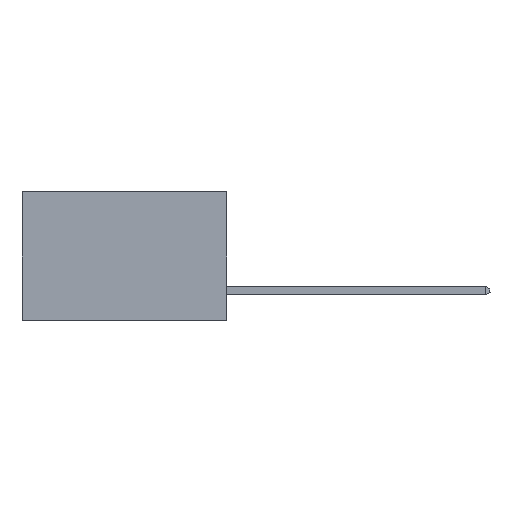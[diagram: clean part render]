
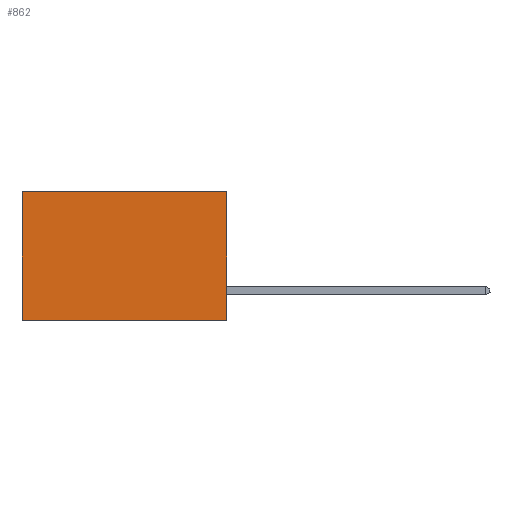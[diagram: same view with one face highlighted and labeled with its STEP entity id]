
A CAD part, left-side view. The second image highlights one B-rep face of the part: STEP entity #862.
In plain terms, the highlighted planar face has unit normal (-1, 0, 0).
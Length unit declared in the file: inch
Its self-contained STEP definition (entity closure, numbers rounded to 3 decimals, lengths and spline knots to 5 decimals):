
#36 = ORIENTED_EDGE ( 'NONE', *, *, #1651, .F. ) ;
#275 = CARTESIAN_POINT ( 'NONE',  ( 0.277, 0.59, 0. ) ) ;
#862 = ADVANCED_FACE ( 'NONE', ( #5057 ), #7052, .F. ) ;
#1097 = VERTEX_POINT ( 'NONE', #275 ) ;
#1651 = EDGE_CURVE ( 'NONE', #5266, #9212, #3417, .T. ) ;
#1673 = EDGE_CURVE ( 'NONE', #7320, #5266, #9046, .T. ) ;
#1677 = CARTESIAN_POINT ( 'NONE',  ( 0.277, 0.59, -0.37 ) ) ;
#1710 = CARTESIAN_POINT ( 'NONE',  ( 0.277, 0.59, -0.37 ) ) ;
#1860 = CARTESIAN_POINT ( 'NONE',  ( 0.277, 0., -0.37 ) ) ;
#2819 = DIRECTION ( 'NONE',  ( 1., 0., 0. ) ) ;
#2960 = CARTESIAN_POINT ( 'NONE',  ( 0.277, 0., 0. ) ) ;
#3206 = CARTESIAN_POINT ( 'NONE',  ( 0.277, 0., -0.37 ) ) ;
#3212 = CARTESIAN_POINT ( 'NONE',  ( 0.277, 0., 0. ) ) ;
#3417 = LINE ( 'NONE', #1860, #7367 ) ;
#4752 = ORIENTED_EDGE ( 'NONE', *, *, #1673, .F. ) ;
#5057 = FACE_OUTER_BOUND ( 'NONE', #7491, .T. ) ;
#5266 = VERTEX_POINT ( 'NONE', #9908 ) ;
#6679 = DIRECTION ( 'NONE',  ( 0., 1., 0. ) ) ;
#6846 = ORIENTED_EDGE ( 'NONE', *, *, #8831, .T. ) ;
#6894 = VECTOR ( 'NONE', #8727, 39.37008 ) ;
#7052 = PLANE ( 'NONE',  #7210 ) ;
#7128 = VECTOR ( 'NONE', #7342, 39.37008 ) ;
#7210 = AXIS2_PLACEMENT_3D ( 'NONE', #9140, #2819, #9097 ) ;
#7320 = VERTEX_POINT ( 'NONE', #2960 ) ;
#7342 = DIRECTION ( 'NONE',  ( 0., 0., -1. ) ) ;
#7367 = VECTOR ( 'NONE', #6679, 39.37008 ) ;
#7491 = EDGE_LOOP ( 'NONE', ( #8580, #36, #4752, #6846 ) ) ;
#7936 = EDGE_CURVE ( 'NONE', #1097, #9212, #8611, .T. ) ;
#8242 = VECTOR ( 'NONE', #8602, 39.37008 ) ;
#8461 = LINE ( 'NONE', #3212, #8242 ) ;
#8580 = ORIENTED_EDGE ( 'NONE', *, *, #7936, .T. ) ;
#8602 = DIRECTION ( 'NONE',  ( 0., 1., 0. ) ) ;
#8611 = LINE ( 'NONE', #1677, #7128 ) ;
#8727 = DIRECTION ( 'NONE',  ( 0., 0., -1. ) ) ;
#8831 = EDGE_CURVE ( 'NONE', #7320, #1097, #8461, .T. ) ;
#9046 = LINE ( 'NONE', #3206, #6894 ) ;
#9097 = DIRECTION ( 'NONE',  ( 0., 0., -1. ) ) ;
#9140 = CARTESIAN_POINT ( 'NONE',  ( 0.277, 0., -0.37 ) ) ;
#9212 = VERTEX_POINT ( 'NONE', #1710 ) ;
#9908 = CARTESIAN_POINT ( 'NONE',  ( 0.277, 0., -0.37 ) ) ;
